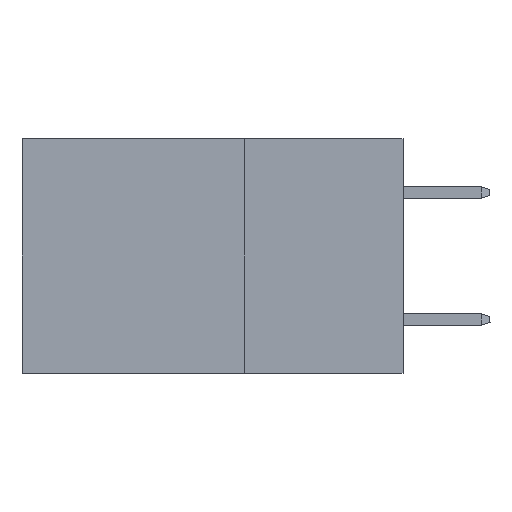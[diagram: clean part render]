
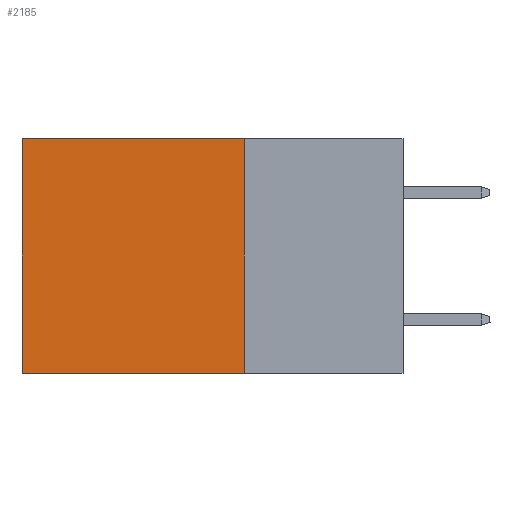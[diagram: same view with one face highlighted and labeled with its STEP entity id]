
A CAD part, left-side view. The second image highlights one B-rep face of the part: STEP entity #2185.
In plain terms, the highlighted planar face has unit normal (-1, 0, 0).
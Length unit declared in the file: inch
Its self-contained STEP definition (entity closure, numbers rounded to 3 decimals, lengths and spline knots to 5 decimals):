
#201 = EDGE_CURVE ( 'NONE', #11626, #14895, #305, .T. ) ;
#211 = VECTOR ( 'NONE', #8009, 39.37008 ) ;
#305 = LINE ( 'NONE', #6808, #211 ) ;
#421 = DIRECTION ( 'NONE',  ( 1., 0., 0. ) ) ;
#1848 = CARTESIAN_POINT ( 'NONE',  ( 0.2875, 0.6, -0.37 ) ) ;
#2185 = ADVANCED_FACE ( 'NONE', ( #11895 ), #15731, .F. ) ;
#3127 = EDGE_CURVE ( 'NONE', #7416, #8187, #5206, .T. ) ;
#3253 = ORIENTED_EDGE ( 'NONE', *, *, #3127, .F. ) ;
#3587 = CARTESIAN_POINT ( 'NONE',  ( 0.2875, 0.25, 0. ) ) ;
#5206 = LINE ( 'NONE', #13986, #16696 ) ;
#5820 = LINE ( 'NONE', #8369, #13004 ) ;
#6775 = EDGE_CURVE ( 'NONE', #14895, #8187, #5820, .T. ) ;
#6808 = CARTESIAN_POINT ( 'NONE',  ( 0.2875, 0.25, 0. ) ) ;
#7145 = VECTOR ( 'NONE', #8664, 39.37008 ) ;
#7416 = VERTEX_POINT ( 'NONE', #12594 ) ;
#7529 = DIRECTION ( 'NONE',  ( 0., 1., 0. ) ) ;
#7664 = CARTESIAN_POINT ( 'NONE',  ( 0.2875, 0.6, 0. ) ) ;
#8009 = DIRECTION ( 'NONE',  ( 0., 1., 0. ) ) ;
#8187 = VERTEX_POINT ( 'NONE', #1848 ) ;
#8369 = CARTESIAN_POINT ( 'NONE',  ( 0.2875, 0.6, 0. ) ) ;
#8664 = DIRECTION ( 'NONE',  ( 0., 0., -1. ) ) ;
#10234 = ORIENTED_EDGE ( 'NONE', *, *, #6775, .T. ) ;
#10862 = DIRECTION ( 'NONE',  ( 0., 0., -1. ) ) ;
#10907 = ORIENTED_EDGE ( 'NONE', *, *, #201, .T. ) ;
#11033 = CARTESIAN_POINT ( 'NONE',  ( 0.2875, 0.25, 0. ) ) ;
#11626 = VERTEX_POINT ( 'NONE', #11033 ) ;
#11895 = FACE_OUTER_BOUND ( 'NONE', #15845, .T. ) ;
#12052 = CARTESIAN_POINT ( 'NONE',  ( 0.2875, 0.25, 0. ) ) ;
#12594 = CARTESIAN_POINT ( 'NONE',  ( 0.2875, 0.25, -0.37 ) ) ;
#12601 = LINE ( 'NONE', #3587, #7145 ) ;
#13004 = VECTOR ( 'NONE', #14755, 39.37008 ) ;
#13384 = AXIS2_PLACEMENT_3D ( 'NONE', #12052, #421, #10862 ) ;
#13803 = EDGE_CURVE ( 'NONE', #11626, #7416, #12601, .T. ) ;
#13986 = CARTESIAN_POINT ( 'NONE',  ( 0.2875, 0.25, -0.37 ) ) ;
#14755 = DIRECTION ( 'NONE',  ( 0., 0., -1. ) ) ;
#14895 = VERTEX_POINT ( 'NONE', #7664 ) ;
#15117 = ORIENTED_EDGE ( 'NONE', *, *, #13803, .F. ) ;
#15731 = PLANE ( 'NONE',  #13384 ) ;
#15845 = EDGE_LOOP ( 'NONE', ( #10234, #3253, #15117, #10907 ) ) ;
#16696 = VECTOR ( 'NONE', #7529, 39.37008 ) ;
